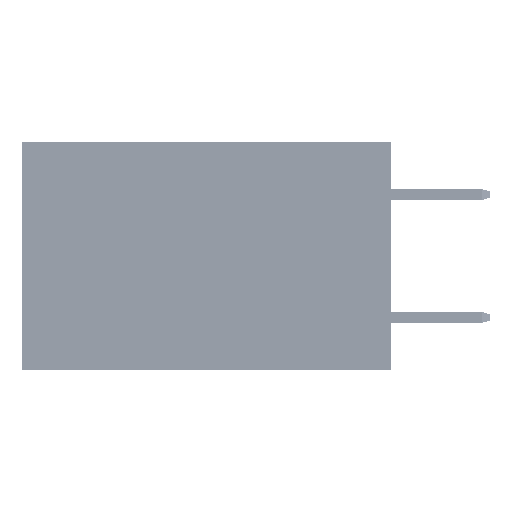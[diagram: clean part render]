
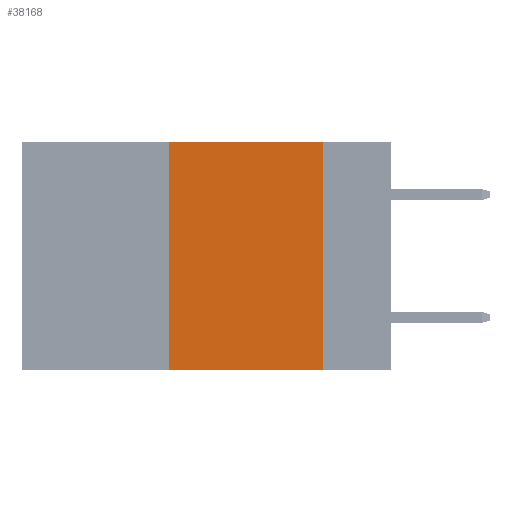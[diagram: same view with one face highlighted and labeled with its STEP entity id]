
A CAD part, left-side view. The second image highlights one B-rep face of the part: STEP entity #38168.
In plain terms, the highlighted planar face has unit normal (-1, 0, 0).
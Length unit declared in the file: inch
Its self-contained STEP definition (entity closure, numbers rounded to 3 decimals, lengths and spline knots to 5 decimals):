
#1387 = VECTOR ( 'NONE', #29951, 39.37008 ) ;
#3100 = EDGE_LOOP ( 'NONE', ( #16889, #20329, #46340, #45338 ) ) ;
#4503 = CARTESIAN_POINT ( 'NONE',  ( 0., 0.11, 0. ) ) ;
#4645 = VERTEX_POINT ( 'NONE', #18981 ) ;
#6175 = EDGE_CURVE ( 'NONE', #27791, #18686, #27917, .T. ) ;
#8514 = DIRECTION ( 'NONE',  ( 0., 0., -1. ) ) ;
#9396 = VECTOR ( 'NONE', #8514, 39.37008 ) ;
#12256 = VERTEX_POINT ( 'NONE', #44164 ) ;
#13189 = CARTESIAN_POINT ( 'NONE',  ( 0., 0.36, 0. ) ) ;
#13810 = LINE ( 'NONE', #29290, #26007 ) ;
#15831 = FACE_OUTER_BOUND ( 'NONE', #3100, .T. ) ;
#16889 = ORIENTED_EDGE ( 'NONE', *, *, #6175, .F. ) ;
#18686 = VERTEX_POINT ( 'NONE', #26027 ) ;
#18981 = CARTESIAN_POINT ( 'NONE',  ( 0., 0.36, 0. ) ) ;
#20018 = AXIS2_PLACEMENT_3D ( 'NONE', #42847, #23439, #39435 ) ;
#20329 = ORIENTED_EDGE ( 'NONE', *, *, #33759, .F. ) ;
#23439 = DIRECTION ( 'NONE',  ( 1., 0., 0. ) ) ;
#25661 = VECTOR ( 'NONE', #44490, 39.37008 ) ;
#26007 = VECTOR ( 'NONE', #49757, 39.37008 ) ;
#26027 = CARTESIAN_POINT ( 'NONE',  ( 0., 0.11, -0.37 ) ) ;
#27416 = EDGE_CURVE ( 'NONE', #12256, #4645, #49139, .T. ) ;
#27791 = VERTEX_POINT ( 'NONE', #4503 ) ;
#27917 = LINE ( 'NONE', #32360, #9396 ) ;
#28477 = CARTESIAN_POINT ( 'NONE',  ( 0., 0.6, -0.37 ) ) ;
#29290 = CARTESIAN_POINT ( 'NONE',  ( 0., 0.6, 0. ) ) ;
#29951 = DIRECTION ( 'NONE',  ( 0., 0., 1. ) ) ;
#32360 = CARTESIAN_POINT ( 'NONE',  ( 0., 0.11, 0. ) ) ;
#33759 = EDGE_CURVE ( 'NONE', #4645, #27791, #13810, .T. ) ;
#35501 = PLANE ( 'NONE',  #20018 ) ;
#35555 = EDGE_CURVE ( 'NONE', #12256, #18686, #48426, .T. ) ;
#38168 = ADVANCED_FACE ( 'NONE', ( #15831 ), #35501, .F. ) ;
#39435 = DIRECTION ( 'NONE',  ( 0., 0., -1. ) ) ;
#42847 = CARTESIAN_POINT ( 'NONE',  ( 0., 0.6, 0. ) ) ;
#44164 = CARTESIAN_POINT ( 'NONE',  ( 0., 0.36, -0.37 ) ) ;
#44490 = DIRECTION ( 'NONE',  ( 0., -1., 0. ) ) ;
#45338 = ORIENTED_EDGE ( 'NONE', *, *, #35555, .T. ) ;
#46340 = ORIENTED_EDGE ( 'NONE', *, *, #27416, .F. ) ;
#48426 = LINE ( 'NONE', #28477, #25661 ) ;
#49139 = LINE ( 'NONE', #13189, #1387 ) ;
#49757 = DIRECTION ( 'NONE',  ( 0., -1., 0. ) ) ;
